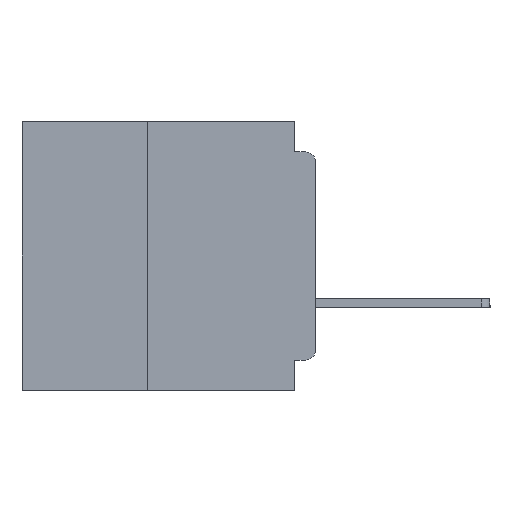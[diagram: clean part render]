
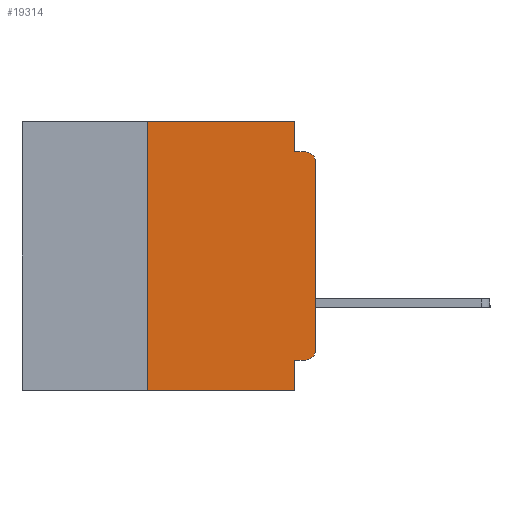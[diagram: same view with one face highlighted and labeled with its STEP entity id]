
A CAD part, left-side view. The second image highlights one B-rep face of the part: STEP entity #19314.
In plain terms, the highlighted planar face has unit normal (-1, 0, 0).
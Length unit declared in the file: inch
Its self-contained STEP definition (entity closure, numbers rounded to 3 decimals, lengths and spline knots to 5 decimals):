
#231 = VERTEX_POINT ( 'NONE', #28147 ) ;
#1090 = ORIENTED_EDGE ( 'NONE', *, *, #15665, .T. ) ;
#1148 = EDGE_CURVE ( 'NONE', #3799, #37503, #20210, .T. ) ;
#2759 = CARTESIAN_POINT ( 'NONE',  ( 0., 0., -0.06 ) ) ;
#2856 = CARTESIAN_POINT ( 'NONE',  ( 0., 0.437, 0. ) ) ;
#2869 = ORIENTED_EDGE ( 'NONE', *, *, #27160, .T. ) ;
#2937 = ORIENTED_EDGE ( 'NONE', *, *, #8450, .T. ) ;
#3484 = VERTEX_POINT ( 'NONE', #14806 ) ;
#3542 = VECTOR ( 'NONE', #19545, 39.37008 ) ;
#3799 = VERTEX_POINT ( 'NONE', #5663 ) ;
#4768 = AXIS2_PLACEMENT_3D ( 'NONE', #48630, #23756, #52697 ) ;
#4785 = VECTOR ( 'NONE', #50090, 39.37008 ) ;
#5501 = VERTEX_POINT ( 'NONE', #2759 ) ;
#5663 = CARTESIAN_POINT ( 'NONE',  ( 0., 0.015, -0.355 ) ) ;
#5818 = CARTESIAN_POINT ( 'NONE',  ( 0., 0.25, 0. ) ) ;
#6889 = CIRCLE ( 'NONE', #39835, 0.015 ) ;
#7039 = PLANE ( 'NONE',  #25984 ) ;
#7206 = LINE ( 'NONE', #40672, #51250 ) ;
#7481 = ORIENTED_EDGE ( 'NONE', *, *, #1148, .F. ) ;
#8450 = EDGE_CURVE ( 'NONE', #48228, #5501, #25355, .T. ) ;
#10890 = CARTESIAN_POINT ( 'NONE',  ( 0., 0., -0.045 ) ) ;
#11611 = VERTEX_POINT ( 'NONE', #5818 ) ;
#11669 = CARTESIAN_POINT ( 'NONE',  ( 0., 0.031, -0.355 ) ) ;
#11688 = DIRECTION ( 'NONE',  ( 0., 1., 0. ) ) ;
#12913 = EDGE_CURVE ( 'NONE', #37503, #35896, #15863, .T. ) ;
#13107 = CARTESIAN_POINT ( 'NONE',  ( 0., 0., -0.355 ) ) ;
#14806 = CARTESIAN_POINT ( 'NONE',  ( 0., 0.25, -0.4 ) ) ;
#15011 = VECTOR ( 'NONE', #27374, 39.37008 ) ;
#15337 = DIRECTION ( 'NONE',  ( 0., 0., -1. ) ) ;
#15380 = CARTESIAN_POINT ( 'NONE',  ( 0., 0.031, -0.4 ) ) ;
#15665 = EDGE_CURVE ( 'NONE', #3484, #35896, #7206, .T. ) ;
#15863 = LINE ( 'NONE', #15380, #3542 ) ;
#17254 = DIRECTION ( 'NONE',  ( 0., 0., 1. ) ) ;
#19314 = ADVANCED_FACE ( 'NONE', ( #39572 ), #7039, .F. ) ;
#19545 = DIRECTION ( 'NONE',  ( 0., 0., -1. ) ) ;
#19926 = DIRECTION ( 'NONE',  ( 0., -1., 0. ) ) ;
#20210 = LINE ( 'NONE', #13107, #41032 ) ;
#20378 = DIRECTION ( 'NONE',  ( 0., 0., -1. ) ) ;
#20922 = CARTESIAN_POINT ( 'NONE',  ( 0., 0.015, -0.34 ) ) ;
#20961 = VERTEX_POINT ( 'NONE', #48496 ) ;
#21220 = EDGE_CURVE ( 'NONE', #3484, #11611, #21240, .T. ) ;
#21240 = LINE ( 'NONE', #50416, #52949 ) ;
#23329 = EDGE_CURVE ( 'NONE', #231, #26896, #48127, .T. ) ;
#23756 = DIRECTION ( 'NONE',  ( -1., 0., 0. ) ) ;
#24010 = ORIENTED_EDGE ( 'NONE', *, *, #38083, .F. ) ;
#24059 = VECTOR ( 'NONE', #49797, 39.37008 ) ;
#24819 = CARTESIAN_POINT ( 'NONE',  ( 0., 0.031, -0.4 ) ) ;
#25069 = DIRECTION ( 'NONE',  ( 0., 0., -1. ) ) ;
#25235 = CARTESIAN_POINT ( 'NONE',  ( 0., 0.437, 0. ) ) ;
#25355 = LINE ( 'NONE', #32256, #24059 ) ;
#25984 = AXIS2_PLACEMENT_3D ( 'NONE', #2856, #40218, #15337 ) ;
#26896 = VERTEX_POINT ( 'NONE', #48192 ) ;
#27160 = EDGE_CURVE ( 'NONE', #3799, #48228, #6889, .T. ) ;
#27253 = ORIENTED_EDGE ( 'NONE', *, *, #35136, .F. ) ;
#27374 = DIRECTION ( 'NONE',  ( 0., -1., 0. ) ) ;
#28147 = CARTESIAN_POINT ( 'NONE',  ( 0., 0.031, -0.045 ) ) ;
#29888 = CIRCLE ( 'NONE', #4768, 0.015 ) ;
#32256 = CARTESIAN_POINT ( 'NONE',  ( 0., 0., 0. ) ) ;
#33958 = LINE ( 'NONE', #25235, #4785 ) ;
#34913 = ORIENTED_EDGE ( 'NONE', *, *, #21220, .F. ) ;
#35136 = EDGE_CURVE ( 'NONE', #20961, #231, #51132, .T. ) ;
#35896 = VERTEX_POINT ( 'NONE', #24819 ) ;
#36683 = EDGE_LOOP ( 'NONE', ( #2937, #51266, #47002, #27253, #24010, #34913, #1090, #49520, #7481, #2869 ) ) ;
#37503 = VERTEX_POINT ( 'NONE', #11669 ) ;
#38083 = EDGE_CURVE ( 'NONE', #11611, #20961, #33958, .T. ) ;
#38876 = VECTOR ( 'NONE', #20378, 39.37008 ) ;
#39572 = FACE_OUTER_BOUND ( 'NONE', #36683, .T. ) ;
#39835 = AXIS2_PLACEMENT_3D ( 'NONE', #20922, #49924, #25069 ) ;
#40218 = DIRECTION ( 'NONE',  ( 1., 0., 0. ) ) ;
#40672 = CARTESIAN_POINT ( 'NONE',  ( 0., 0.437, -0.4 ) ) ;
#41032 = VECTOR ( 'NONE', #11688, 39.37008 ) ;
#46670 = EDGE_CURVE ( 'NONE', #5501, #26896, #29888, .T. ) ;
#47002 = ORIENTED_EDGE ( 'NONE', *, *, #23329, .F. ) ;
#48127 = LINE ( 'NONE', #10890, #15011 ) ;
#48192 = CARTESIAN_POINT ( 'NONE',  ( 0., 0.015, -0.045 ) ) ;
#48228 = VERTEX_POINT ( 'NONE', #50252 ) ;
#48496 = CARTESIAN_POINT ( 'NONE',  ( 0., 0.031, 0. ) ) ;
#48630 = CARTESIAN_POINT ( 'NONE',  ( 0., 0.015, -0.06 ) ) ;
#49404 = CARTESIAN_POINT ( 'NONE',  ( 0., 0.031, 0. ) ) ;
#49520 = ORIENTED_EDGE ( 'NONE', *, *, #12913, .F. ) ;
#49797 = DIRECTION ( 'NONE',  ( 0., 0., 1. ) ) ;
#49924 = DIRECTION ( 'NONE',  ( -1., 0., 0. ) ) ;
#50090 = DIRECTION ( 'NONE',  ( 0., -1., 0. ) ) ;
#50252 = CARTESIAN_POINT ( 'NONE',  ( 0., 0., -0.34 ) ) ;
#50416 = CARTESIAN_POINT ( 'NONE',  ( 0., 0.25, -0.4 ) ) ;
#51132 = LINE ( 'NONE', #49404, #38876 ) ;
#51250 = VECTOR ( 'NONE', #19926, 39.37008 ) ;
#51266 = ORIENTED_EDGE ( 'NONE', *, *, #46670, .T. ) ;
#52697 = DIRECTION ( 'NONE',  ( 0., 0., -1. ) ) ;
#52949 = VECTOR ( 'NONE', #17254, 39.37008 ) ;
